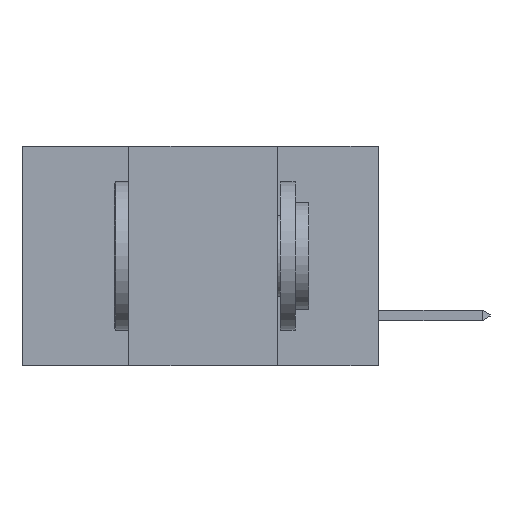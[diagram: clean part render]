
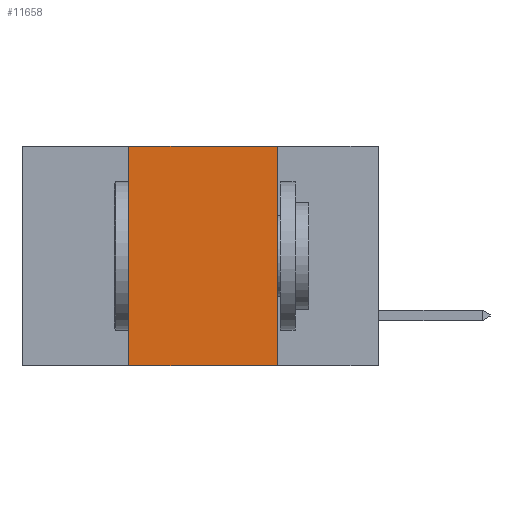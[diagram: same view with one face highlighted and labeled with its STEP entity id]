
A CAD part, left-side view. The second image highlights one B-rep face of the part: STEP entity #11658.
In plain terms, the highlighted planar face has unit normal (-1, 0, 0).
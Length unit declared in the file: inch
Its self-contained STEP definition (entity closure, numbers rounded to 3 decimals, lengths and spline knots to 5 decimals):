
#58 = DIRECTION ( 'NONE',  ( 0., -1., 0. ) ) ;
#288 = VERTEX_POINT ( 'NONE', #9132 ) ;
#416 = DIRECTION ( 'NONE',  ( 0., 0., -1. ) ) ;
#994 = CARTESIAN_POINT ( 'NONE',  ( 0., 0.42, -0.37 ) ) ;
#1022 = VERTEX_POINT ( 'NONE', #8058 ) ;
#1064 = DIRECTION ( 'NONE',  ( 0., 0., 1. ) ) ;
#1139 = CARTESIAN_POINT ( 'NONE',  ( 0., 0.6, 0. ) ) ;
#1705 = VECTOR ( 'NONE', #1064, 39.37008 ) ;
#2224 = LINE ( 'NONE', #12233, #12470 ) ;
#2421 = LINE ( 'NONE', #994, #1705 ) ;
#3020 = ORIENTED_EDGE ( 'NONE', *, *, #7070, .F. ) ;
#3225 = ORIENTED_EDGE ( 'NONE', *, *, #6412, .F. ) ;
#3370 = ORIENTED_EDGE ( 'NONE', *, *, #5726, .F. ) ;
#3465 = ORIENTED_EDGE ( 'NONE', *, *, #5025, .T. ) ;
#4073 = VERTEX_POINT ( 'NONE', #7958 ) ;
#4425 = VECTOR ( 'NONE', #4709, 39.37008 ) ;
#4709 = DIRECTION ( 'NONE',  ( 0., -1., 0. ) ) ;
#4759 = CARTESIAN_POINT ( 'NONE',  ( 0., 0.6, -0.37 ) ) ;
#5025 = EDGE_CURVE ( 'NONE', #288, #9904, #11950, .T. ) ;
#5363 = PLANE ( 'NONE',  #9060 ) ;
#5454 = DIRECTION ( 'NONE',  ( 0., 0., -1. ) ) ;
#5726 = EDGE_CURVE ( 'NONE', #288, #4073, #2421, .T. ) ;
#5809 = CARTESIAN_POINT ( 'NONE',  ( 0., 0.17, -0.37 ) ) ;
#5821 = CARTESIAN_POINT ( 'NONE',  ( 0., 0.17, -0.37 ) ) ;
#6412 = EDGE_CURVE ( 'NONE', #4073, #1022, #2224, .T. ) ;
#7003 = EDGE_LOOP ( 'NONE', ( #3020, #3225, #3370, #3465 ) ) ;
#7070 = EDGE_CURVE ( 'NONE', #1022, #9904, #11457, .T. ) ;
#7958 = CARTESIAN_POINT ( 'NONE',  ( 0., 0.42, 0. ) ) ;
#8058 = CARTESIAN_POINT ( 'NONE',  ( 0., 0.17, 0. ) ) ;
#8998 = VECTOR ( 'NONE', #416, 39.37008 ) ;
#9060 = AXIS2_PLACEMENT_3D ( 'NONE', #1139, #11312, #5454 ) ;
#9132 = CARTESIAN_POINT ( 'NONE',  ( 0., 0.42, -0.37 ) ) ;
#9904 = VERTEX_POINT ( 'NONE', #5809 ) ;
#10816 = FACE_OUTER_BOUND ( 'NONE', #7003, .T. ) ;
#11312 = DIRECTION ( 'NONE',  ( 1., 0., 0. ) ) ;
#11457 = LINE ( 'NONE', #5821, #8998 ) ;
#11658 = ADVANCED_FACE ( 'NONE', ( #10816 ), #5363, .F. ) ;
#11950 = LINE ( 'NONE', #4759, #4425 ) ;
#12233 = CARTESIAN_POINT ( 'NONE',  ( 0., 0.6, 0. ) ) ;
#12470 = VECTOR ( 'NONE', #58, 39.37008 ) ;
